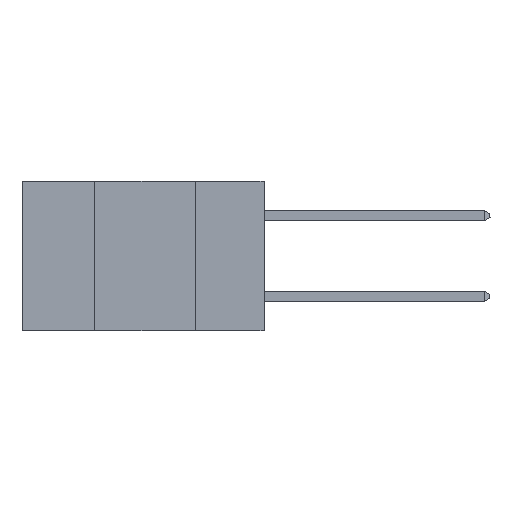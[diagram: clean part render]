
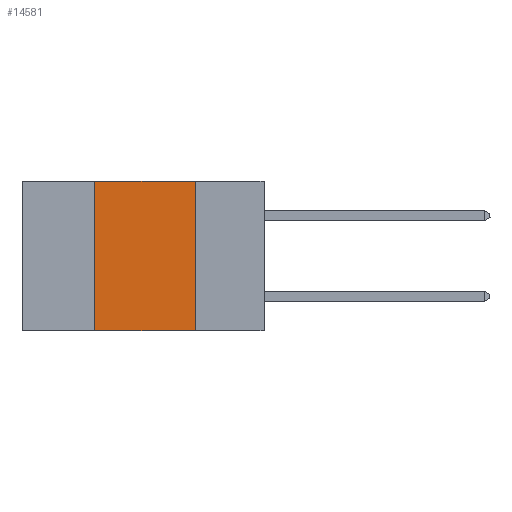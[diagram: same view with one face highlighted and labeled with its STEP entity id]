
A CAD part, left-side view. The second image highlights one B-rep face of the part: STEP entity #14581.
In plain terms, the highlighted planar face has unit normal (-1, 0, 0).
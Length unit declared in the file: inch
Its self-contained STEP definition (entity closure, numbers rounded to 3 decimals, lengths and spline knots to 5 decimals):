
#52 = VERTEX_POINT ( 'NONE', #3469 ) ;
#183 = CARTESIAN_POINT ( 'NONE',  ( 0., 0.6, 0. ) ) ;
#1146 = EDGE_CURVE ( 'NONE', #1880, #2588, #16377, .T. ) ;
#1296 = EDGE_LOOP ( 'NONE', ( #13330, #14672, #16652, #4285 ) ) ;
#1880 = VERTEX_POINT ( 'NONE', #16786 ) ;
#1993 = CARTESIAN_POINT ( 'NONE',  ( 0., 0.42, -0.37 ) ) ;
#2041 = LINE ( 'NONE', #22628, #16830 ) ;
#2588 = VERTEX_POINT ( 'NONE', #4419 ) ;
#2989 = EDGE_CURVE ( 'NONE', #12102, #2588, #14691, .T. ) ;
#3469 = CARTESIAN_POINT ( 'NONE',  ( 0., 0.42, 0. ) ) ;
#4285 = ORIENTED_EDGE ( 'NONE', *, *, #2989, .T. ) ;
#4419 = CARTESIAN_POINT ( 'NONE',  ( 0., 0.17, -0.37 ) ) ;
#4839 = VECTOR ( 'NONE', #20502, 39.37008 ) ;
#4881 = EDGE_CURVE ( 'NONE', #12102, #52, #2041, .T. ) ;
#5995 = EDGE_CURVE ( 'NONE', #52, #1880, #14765, .T. ) ;
#7617 = FACE_OUTER_BOUND ( 'NONE', #1296, .T. ) ;
#9169 = PLANE ( 'NONE',  #13263 ) ;
#10454 = DIRECTION ( 'NONE',  ( 0., 0., -1. ) ) ;
#11651 = CARTESIAN_POINT ( 'NONE',  ( 0., 0.6, 0. ) ) ;
#12102 = VERTEX_POINT ( 'NONE', #1993 ) ;
#13263 = AXIS2_PLACEMENT_3D ( 'NONE', #11651, #15226, #19494 ) ;
#13330 = ORIENTED_EDGE ( 'NONE', *, *, #1146, .F. ) ;
#14581 = ADVANCED_FACE ( 'NONE', ( #7617 ), #9169, .F. ) ;
#14672 = ORIENTED_EDGE ( 'NONE', *, *, #5995, .F. ) ;
#14691 = LINE ( 'NONE', #24561, #4839 ) ;
#14765 = LINE ( 'NONE', #183, #22870 ) ;
#15226 = DIRECTION ( 'NONE',  ( 1., 0., 0. ) ) ;
#16025 = DIRECTION ( 'NONE',  ( 0., -1., 0. ) ) ;
#16377 = LINE ( 'NONE', #16378, #18529 ) ;
#16378 = CARTESIAN_POINT ( 'NONE',  ( 0., 0.17, 0. ) ) ;
#16652 = ORIENTED_EDGE ( 'NONE', *, *, #4881, .F. ) ;
#16786 = CARTESIAN_POINT ( 'NONE',  ( 0., 0.17, 0. ) ) ;
#16830 = VECTOR ( 'NONE', #22457, 39.37008 ) ;
#18529 = VECTOR ( 'NONE', #10454, 39.37008 ) ;
#19494 = DIRECTION ( 'NONE',  ( 0., 0., -1. ) ) ;
#20502 = DIRECTION ( 'NONE',  ( 0., -1., 0. ) ) ;
#22457 = DIRECTION ( 'NONE',  ( 0., 0., 1. ) ) ;
#22628 = CARTESIAN_POINT ( 'NONE',  ( 0., 0.42, 0. ) ) ;
#22870 = VECTOR ( 'NONE', #16025, 39.37008 ) ;
#24561 = CARTESIAN_POINT ( 'NONE',  ( 0., 0.6, -0.37 ) ) ;
